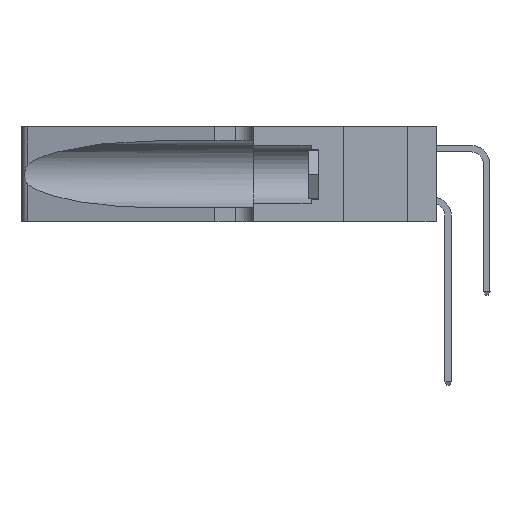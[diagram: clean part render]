
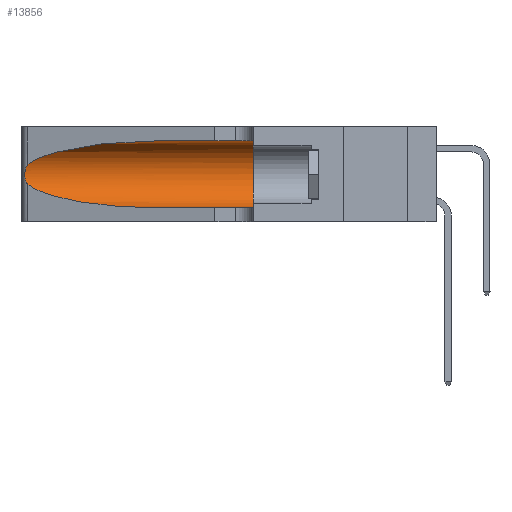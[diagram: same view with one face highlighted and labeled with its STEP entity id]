
A CAD part, left-side view. The second image highlights one B-rep face of the part: STEP entity #13856.
In plain terms, the highlighted cylindrical face has radius 3.308 mm (diameter 6.617 mm), a partial arc.
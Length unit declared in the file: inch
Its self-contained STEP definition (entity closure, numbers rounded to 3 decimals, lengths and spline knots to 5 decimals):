
#382 = CARTESIAN_POINT ( 'NONE',  ( 0.26075, 1.23896, 0.178 ) ) ;
#1024 = AXIS2_PLACEMENT_3D ( 'NONE', #30383, #12050, #11801 ) ;
#1521 = LINE ( 'NONE', #34564, #7349 ) ;
#1886 = ORIENTED_EDGE ( 'NONE', *, *, #38204, .F. ) ;
#3432 = DIRECTION ( 'NONE',  ( 0., -1., 0. ) ) ;
#3433 = EDGE_CURVE ( 'NONE', #15240, #31103, #14104, .T. ) ;
#3747 = CARTESIAN_POINT ( 'NONE',  ( 0.25555, 1.22993, 0.14849 ) ) ;
#3880 = CARTESIAN_POINT ( 'NONE',  ( 0.25487, 1.22718, 0.14631 ) ) ;
#5488 = VERTEX_POINT ( 'NONE', #24933 ) ;
#5854 = ORIENTED_EDGE ( 'NONE', *, *, #18831, .T. ) ;
#6153 = CARTESIAN_POINT ( 'NONE',  ( 0.1305, 1.61858, 0.31525 ) ) ;
#6469 = CARTESIAN_POINT ( 'NONE',  ( 0.25789, 1.23486, 0.15765 ) ) ;
#7349 = VECTOR ( 'NONE', #16473, 39.37008 ) ;
#7351 = CARTESIAN_POINT ( 'NONE',  ( 0.1305, 0.35, 0.31525 ) ) ;
#7607 = ORIENTED_EDGE ( 'NONE', *, *, #25480, .F. ) ;
#8277 = VERTEX_POINT ( 'NONE', #17929 ) ;
#9895 =( BOUNDED_CURVE ( )  B_SPLINE_CURVE ( 3, ( #23632, #27176, #36180, #20807 ),
 .UNSPECIFIED., .F., .T. ) 
 B_SPLINE_CURVE_WITH_KNOTS ( ( 4, 4 ),
 ( 3.44316, 4.71239 ),
 .UNSPECIFIED. ) 
 CURVE ( )  GEOMETRIC_REPRESENTATION_ITEM ( )  RATIONAL_B_SPLINE_CURVE ( ( 1., 0.87, 0.87, 1. ) ) 
 REPRESENTATION_ITEM ( '' )  );
#10139 = CARTESIAN_POINT ( 'NONE',  ( 0.26017, 1.23833, 0.17102 ) ) ;
#10260 = FACE_OUTER_BOUND ( 'NONE', #27264, .T. ) ;
#10692 = CARTESIAN_POINT ( 'NONE',  ( 0.1305, 0.35, 0.185 ) ) ;
#11801 = DIRECTION ( 'NONE',  ( 0., 0., -1. ) ) ;
#12050 = DIRECTION ( 'NONE',  ( 0., -1., 0. ) ) ;
#12977 = CARTESIAN_POINT ( 'NONE',  ( 0.25487, 1.22718, 0.22369 ) ) ;
#13244 = CARTESIAN_POINT ( 'NONE',  ( 0.25639, 1.23186, 0.15144 ) ) ;
#13522 = VERTEX_POINT ( 'NONE', #35182 ) ;
#13856 = ADVANCED_FACE ( 'NONE', ( #10260 ), #20900, .F. ) ;
#14104 =( BOUNDED_CURVE ( )  B_SPLINE_CURVE ( 3, ( #28433, #19317, #31549, #25419 ),
 .UNSPECIFIED., .F., .F. ) 
 B_SPLINE_CURVE_WITH_KNOTS ( ( 4, 4 ),
 ( 1.5708, 2.84003 ),
 .UNSPECIFIED. ) 
 CURVE ( )  GEOMETRIC_REPRESENTATION_ITEM ( )  RATIONAL_B_SPLINE_CURVE ( ( 1., 0.87, 0.87, 1. ) ) 
 REPRESENTATION_ITEM ( '' )  );
#15240 = VERTEX_POINT ( 'NONE', #25352 ) ;
#16473 = DIRECTION ( 'NONE',  ( 0., -1., 0. ) ) ;
#16850 = CIRCLE ( 'NONE', #27579, 0.13025 ) ;
#17929 = CARTESIAN_POINT ( 'NONE',  ( 0.1305, 0.35, 0.05475 ) ) ;
#18332 = ORIENTED_EDGE ( 'NONE', *, *, #27802, .T. ) ;
#18831 = EDGE_CURVE ( 'NONE', #31103, #13522, #22018, .T. ) ;
#19317 = CARTESIAN_POINT ( 'NONE',  ( 0.18966, 0.96281, 0.31525 ) ) ;
#19482 = CARTESIAN_POINT ( 'NONE',  ( 0.26075, 1.23896, 0.19203 ) ) ;
#20807 = CARTESIAN_POINT ( 'NONE',  ( 0.1305, 0.72297, 0.05475 ) ) ;
#20900 = CYLINDRICAL_SURFACE ( 'NONE', #1024, 0.13025 ) ;
#22018 = B_SPLINE_CURVE_WITH_KNOTS ( 'NONE', 3,
 ( #12977, #34986, #25163, #38071, #34723, #31311, #19482, #382, #10139, #31855, #6469, #13244, #3747, #3880 ),
 .UNSPECIFIED., .F., .F.,
 ( 4, 2, 2, 2, 2, 2, 4 ),
 ( 0., 0.00027, 0.00053, 0.00107, 0.0016, 0.00187, 0.00214 ),
 .UNSPECIFIED. ) ;
#22856 = DIRECTION ( 'NONE',  ( 0., 0., 1. ) ) ;
#23632 = CARTESIAN_POINT ( 'NONE',  ( 0.25487, 1.22718, 0.14631 ) ) ;
#24373 = ORIENTED_EDGE ( 'NONE', *, *, #3433, .T. ) ;
#24933 = CARTESIAN_POINT ( 'NONE',  ( 0.1305, 0.72297, 0.05475 ) ) ;
#25163 = CARTESIAN_POINT ( 'NONE',  ( 0.25639, 1.23184, 0.21858 ) ) ;
#25352 = CARTESIAN_POINT ( 'NONE',  ( 0.1305, 0.72297, 0.31525 ) ) ;
#25419 = CARTESIAN_POINT ( 'NONE',  ( 0.25487, 1.22718, 0.22369 ) ) ;
#25480 = EDGE_CURVE ( 'NONE', #15240, #28568, #32554, .T. ) ;
#27029 = ORIENTED_EDGE ( 'NONE', *, *, #36351, .T. ) ;
#27176 = CARTESIAN_POINT ( 'NONE',  ( 0.2373, 1.15595, 0.08982 ) ) ;
#27264 = EDGE_LOOP ( 'NONE', ( #24373, #5854, #27029, #18332, #1886, #7607 ) ) ;
#27579 = AXIS2_PLACEMENT_3D ( 'NONE', #10692, #28889, #22856 ) ;
#27649 = VECTOR ( 'NONE', #3432, 39.37008 ) ;
#27802 = EDGE_CURVE ( 'NONE', #5488, #8277, #1521, .T. ) ;
#28433 = CARTESIAN_POINT ( 'NONE',  ( 0.1305, 0.72297, 0.31525 ) ) ;
#28568 = VERTEX_POINT ( 'NONE', #7351 ) ;
#28889 = DIRECTION ( 'NONE',  ( 0., 1., 0. ) ) ;
#30383 = CARTESIAN_POINT ( 'NONE',  ( 0.1305, 1.61858, 0.185 ) ) ;
#31103 = VERTEX_POINT ( 'NONE', #31775 ) ;
#31311 = CARTESIAN_POINT ( 'NONE',  ( 0.26018, 1.23835, 0.19895 ) ) ;
#31549 = CARTESIAN_POINT ( 'NONE',  ( 0.2373, 1.15595, 0.28018 ) ) ;
#31775 = CARTESIAN_POINT ( 'NONE',  ( 0.25487, 1.22718, 0.22369 ) ) ;
#31855 = CARTESIAN_POINT ( 'NONE',  ( 0.25856, 1.23593, 0.16098 ) ) ;
#32554 = LINE ( 'NONE', #6153, #27649 ) ;
#34564 = CARTESIAN_POINT ( 'NONE',  ( 0.1305, 1.61858, 0.05475 ) ) ;
#34723 = CARTESIAN_POINT ( 'NONE',  ( 0.25854, 1.2359, 0.20912 ) ) ;
#34986 = CARTESIAN_POINT ( 'NONE',  ( 0.25555, 1.22994, 0.2215 ) ) ;
#35182 = CARTESIAN_POINT ( 'NONE',  ( 0.25487, 1.22718, 0.14631 ) ) ;
#36180 = CARTESIAN_POINT ( 'NONE',  ( 0.18966, 0.96281, 0.05475 ) ) ;
#36351 = EDGE_CURVE ( 'NONE', #13522, #5488, #9895, .T. ) ;
#38071 = CARTESIAN_POINT ( 'NONE',  ( 0.25787, 1.23484, 0.2124 ) ) ;
#38204 = EDGE_CURVE ( 'NONE', #28568, #8277, #16850, .T. ) ;
